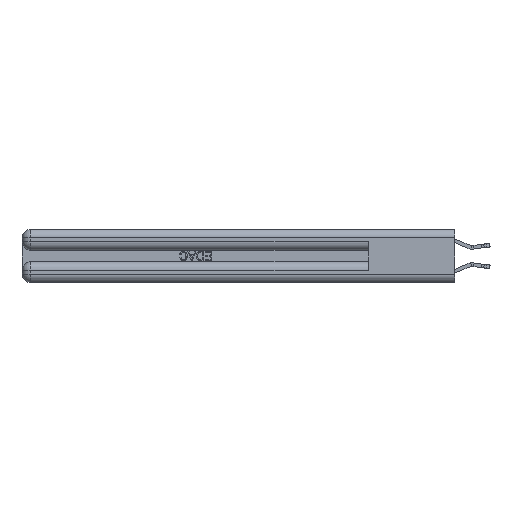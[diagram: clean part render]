
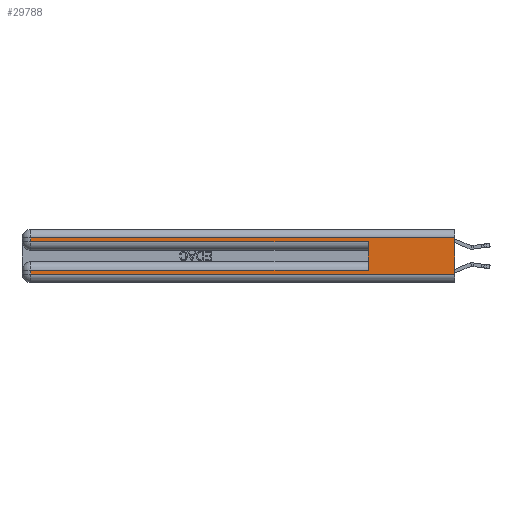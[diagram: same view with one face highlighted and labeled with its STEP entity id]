
A CAD part, left-side view. The second image highlights one B-rep face of the part: STEP entity #29788.
In plain terms, the highlighted planar face has unit normal (-1, 0, 0).
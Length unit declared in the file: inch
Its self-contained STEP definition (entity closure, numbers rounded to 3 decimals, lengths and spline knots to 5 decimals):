
#67 = CARTESIAN_POINT ( 'NONE',  ( 0., 0., 0.285 ) ) ;
#1126 = EDGE_CURVE ( 'NONE', #20619, #11949, #24257, .T. ) ;
#1235 = ORIENTED_EDGE ( 'NONE', *, *, #10985, .T. ) ;
#1592 = EDGE_CURVE ( 'NONE', #13091, #13539, #17582, .T. ) ;
#2240 = CARTESIAN_POINT ( 'NONE',  ( 0., 2.94, 0.285 ) ) ;
#4069 = DIRECTION ( 'NONE',  ( 0., 0., -1. ) ) ;
#4346 = CARTESIAN_POINT ( 'NONE',  ( 0., 2.94, 0.37 ) ) ;
#4357 = DIRECTION ( 'NONE',  ( 0., 0., 1. ) ) ;
#4420 = DIRECTION ( 'NONE',  ( 1., 0., 0. ) ) ;
#4511 = VERTEX_POINT ( 'NONE', #2240 ) ;
#5073 = FACE_OUTER_BOUND ( 'NONE', #31206, .T. ) ;
#5151 = VECTOR ( 'NONE', #4069, 39.37008 ) ;
#5198 = LINE ( 'NONE', #8010, #10996 ) ;
#6355 = CARTESIAN_POINT ( 'NONE',  ( 0., 0.6, 0.085 ) ) ;
#7222 = ORIENTED_EDGE ( 'NONE', *, *, #31765, .T. ) ;
#7331 = ORIENTED_EDGE ( 'NONE', *, *, #23682, .T. ) ;
#7718 = CARTESIAN_POINT ( 'NONE',  ( 0., 0., 0.37 ) ) ;
#8010 = CARTESIAN_POINT ( 'NONE',  ( 0., 0., 0.06 ) ) ;
#8371 = ORIENTED_EDGE ( 'NONE', *, *, #1592, .T. ) ;
#9032 = VERTEX_POINT ( 'NONE', #12270 ) ;
#9662 = VERTEX_POINT ( 'NONE', #11190 ) ;
#9830 = LINE ( 'NONE', #4346, #26086 ) ;
#10170 = ORIENTED_EDGE ( 'NONE', *, *, #24768, .T. ) ;
#10985 = EDGE_CURVE ( 'NONE', #4511, #26460, #22861, .T. ) ;
#10996 = VECTOR ( 'NONE', #12707, 39.37008 ) ;
#11190 = CARTESIAN_POINT ( 'NONE',  ( 0., 0., 0.06 ) ) ;
#11330 = CARTESIAN_POINT ( 'NONE',  ( 0., 2.94, 0.37 ) ) ;
#11949 = VERTEX_POINT ( 'NONE', #30080 ) ;
#12270 = CARTESIAN_POINT ( 'NONE',  ( 0., 2.94, 0.06 ) ) ;
#12707 = DIRECTION ( 'NONE',  ( 0., -1., 0. ) ) ;
#12850 = VECTOR ( 'NONE', #26296, 39.37008 ) ;
#13091 = VERTEX_POINT ( 'NONE', #13527 ) ;
#13527 = CARTESIAN_POINT ( 'NONE',  ( 0., 0., 0.31 ) ) ;
#13539 = VERTEX_POINT ( 'NONE', #15104 ) ;
#14568 = EDGE_CURVE ( 'NONE', #20619, #26460, #27145, .T. ) ;
#15006 = DIRECTION ( 'NONE',  ( 0., 0., -1. ) ) ;
#15104 = CARTESIAN_POINT ( 'NONE',  ( 0., 2.94, 0.31 ) ) ;
#16805 = DIRECTION ( 'NONE',  ( 0., 1., 0. ) ) ;
#17582 = LINE ( 'NONE', #30522, #32523 ) ;
#18371 = DIRECTION ( 'NONE',  ( 0., -1., 0. ) ) ;
#19821 = CARTESIAN_POINT ( 'NONE',  ( 0., 0.6, 0.145 ) ) ;
#20619 = VERTEX_POINT ( 'NONE', #6355 ) ;
#21129 = VECTOR ( 'NONE', #16805, 39.37008 ) ;
#21135 = ORIENTED_EDGE ( 'NONE', *, *, #14568, .F. ) ;
#22861 = LINE ( 'NONE', #67, #23056 ) ;
#22942 = ORIENTED_EDGE ( 'NONE', *, *, #24417, .F. ) ;
#23056 = VECTOR ( 'NONE', #18371, 39.37008 ) ;
#23152 = VECTOR ( 'NONE', #4357, 39.37008 ) ;
#23682 = EDGE_CURVE ( 'NONE', #11949, #9032, #28788, .T. ) ;
#24028 = CARTESIAN_POINT ( 'NONE',  ( 0., 0., 0.37 ) ) ;
#24257 = LINE ( 'NONE', #26925, #21129 ) ;
#24417 = EDGE_CURVE ( 'NONE', #13091, #9662, #29009, .T. ) ;
#24768 = EDGE_CURVE ( 'NONE', #9032, #9662, #5198, .T. ) ;
#25362 = DIRECTION ( 'NONE',  ( 0., 1., 0. ) ) ;
#26086 = VECTOR ( 'NONE', #15006, 39.37008 ) ;
#26296 = DIRECTION ( 'NONE',  ( 0., 0., -1. ) ) ;
#26460 = VERTEX_POINT ( 'NONE', #30446 ) ;
#26925 = CARTESIAN_POINT ( 'NONE',  ( 0., 0., 0.085 ) ) ;
#27145 = LINE ( 'NONE', #19821, #23152 ) ;
#28788 = LINE ( 'NONE', #11330, #12850 ) ;
#29009 = LINE ( 'NONE', #24028, #5151 ) ;
#29761 = AXIS2_PLACEMENT_3D ( 'NONE', #7718, #4420, #32846 ) ;
#29788 = ADVANCED_FACE ( 'NONE', ( #5073 ), #30514, .F. ) ;
#30080 = CARTESIAN_POINT ( 'NONE',  ( 0., 2.94, 0.085 ) ) ;
#30446 = CARTESIAN_POINT ( 'NONE',  ( 0., 0.6, 0.285 ) ) ;
#30514 = PLANE ( 'NONE',  #29761 ) ;
#30522 = CARTESIAN_POINT ( 'NONE',  ( 0., 0., 0.31 ) ) ;
#31206 = EDGE_LOOP ( 'NONE', ( #22942, #8371, #7222, #1235, #21135, #32039, #7331, #10170 ) ) ;
#31765 = EDGE_CURVE ( 'NONE', #13539, #4511, #9830, .T. ) ;
#32039 = ORIENTED_EDGE ( 'NONE', *, *, #1126, .T. ) ;
#32523 = VECTOR ( 'NONE', #25362, 39.37008 ) ;
#32846 = DIRECTION ( 'NONE',  ( 0., 0., -1. ) ) ;
